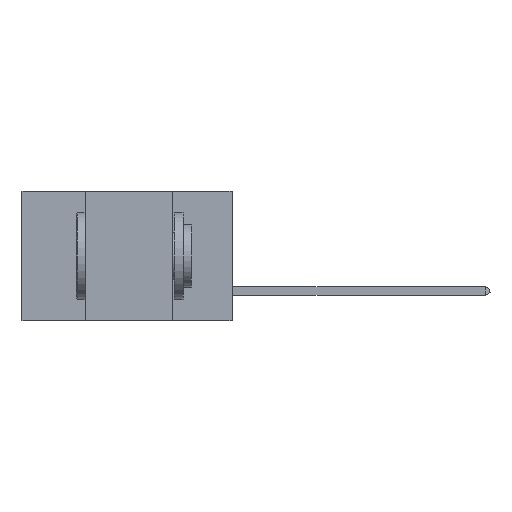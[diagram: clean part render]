
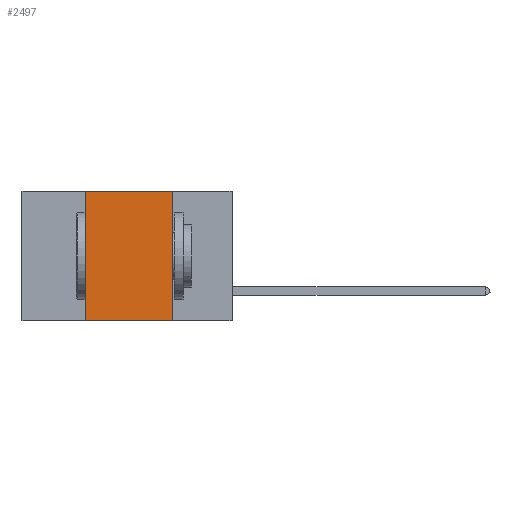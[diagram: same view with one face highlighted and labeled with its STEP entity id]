
A CAD part, left-side view. The second image highlights one B-rep face of the part: STEP entity #2497.
In plain terms, the highlighted planar face has unit normal (-1, 0, 0).
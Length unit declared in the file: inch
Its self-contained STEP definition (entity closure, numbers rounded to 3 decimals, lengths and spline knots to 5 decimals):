
#1298 = VECTOR ( 'NONE', #40982, 39.37008 ) ;
#1430 = CARTESIAN_POINT ( 'NONE',  ( 0., 0.42, -0.37 ) ) ;
#1658 = LINE ( 'NONE', #37571, #38287 ) ;
#2497 = ADVANCED_FACE ( 'NONE', ( #44812 ), #22218, .F. ) ;
#7441 = LINE ( 'NONE', #8745, #28519 ) ;
#8273 = DIRECTION ( 'NONE',  ( 0., 0., -1. ) ) ;
#8745 = CARTESIAN_POINT ( 'NONE',  ( 0., 0.42, 0. ) ) ;
#10322 = CARTESIAN_POINT ( 'NONE',  ( 0., 0.17, -0.37 ) ) ;
#10858 = AXIS2_PLACEMENT_3D ( 'NONE', #22518, #29777, #8273 ) ;
#11457 = LINE ( 'NONE', #18880, #38081 ) ;
#14140 = ORIENTED_EDGE ( 'NONE', *, *, #36249, .T. ) ;
#14708 = CARTESIAN_POINT ( 'NONE',  ( 0., 0.17, 0. ) ) ;
#16142 = CARTESIAN_POINT ( 'NONE',  ( 0., 0.6, 0. ) ) ;
#16200 = ORIENTED_EDGE ( 'NONE', *, *, #24786, .F. ) ;
#18600 = EDGE_CURVE ( 'NONE', #21537, #45144, #7441, .T. ) ;
#18880 = CARTESIAN_POINT ( 'NONE',  ( 0., 0.17, 0. ) ) ;
#20288 = ORIENTED_EDGE ( 'NONE', *, *, #18600, .F. ) ;
#21537 = VERTEX_POINT ( 'NONE', #1430 ) ;
#22043 = EDGE_LOOP ( 'NONE', ( #34474, #16200, #20288, #14140 ) ) ;
#22218 = PLANE ( 'NONE',  #10858 ) ;
#22518 = CARTESIAN_POINT ( 'NONE',  ( 0., 0.6, 0. ) ) ;
#24786 = EDGE_CURVE ( 'NONE', #45144, #43732, #25734, .T. ) ;
#25734 = LINE ( 'NONE', #16142, #1298 ) ;
#28519 = VECTOR ( 'NONE', #33864, 39.37008 ) ;
#29777 = DIRECTION ( 'NONE',  ( 1., 0., 0. ) ) ;
#30413 = DIRECTION ( 'NONE',  ( 0., -1., 0. ) ) ;
#33864 = DIRECTION ( 'NONE',  ( 0., 0., 1. ) ) ;
#34474 = ORIENTED_EDGE ( 'NONE', *, *, #41879, .F. ) ;
#36249 = EDGE_CURVE ( 'NONE', #21537, #42120, #1658, .T. ) ;
#37181 = DIRECTION ( 'NONE',  ( 0., 0., -1. ) ) ;
#37571 = CARTESIAN_POINT ( 'NONE',  ( 0., 0.6, -0.37 ) ) ;
#37757 = CARTESIAN_POINT ( 'NONE',  ( 0., 0.42, 0. ) ) ;
#38081 = VECTOR ( 'NONE', #37181, 39.37008 ) ;
#38287 = VECTOR ( 'NONE', #30413, 39.37008 ) ;
#40982 = DIRECTION ( 'NONE',  ( 0., -1., 0. ) ) ;
#41879 = EDGE_CURVE ( 'NONE', #43732, #42120, #11457, .T. ) ;
#42120 = VERTEX_POINT ( 'NONE', #10322 ) ;
#43732 = VERTEX_POINT ( 'NONE', #14708 ) ;
#44812 = FACE_OUTER_BOUND ( 'NONE', #22043, .T. ) ;
#45144 = VERTEX_POINT ( 'NONE', #37757 ) ;
